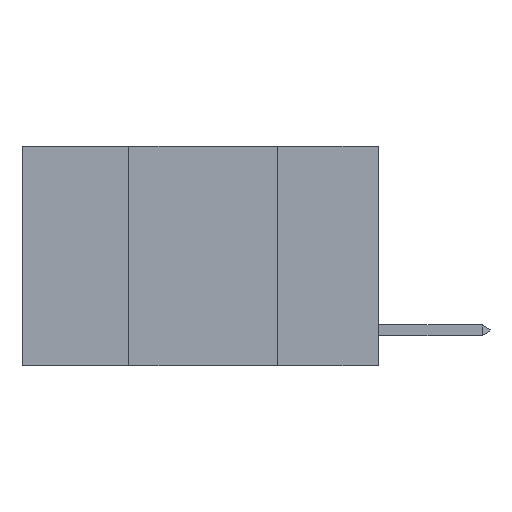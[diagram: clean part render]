
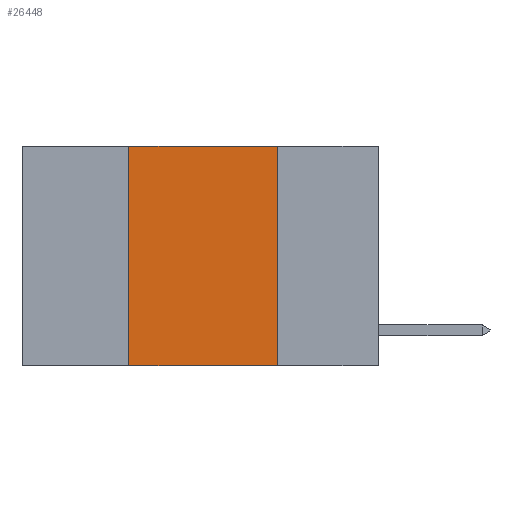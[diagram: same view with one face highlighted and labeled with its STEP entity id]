
A CAD part, left-side view. The second image highlights one B-rep face of the part: STEP entity #26448.
In plain terms, the highlighted planar face has unit normal (-1, 0, 0).
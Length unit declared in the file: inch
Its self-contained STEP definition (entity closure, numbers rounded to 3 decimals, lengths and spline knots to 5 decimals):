
#1099 = DIRECTION ( 'NONE',  ( 0., 0., -1. ) ) ;
#2393 = VERTEX_POINT ( 'NONE', #9922 ) ;
#3205 = CARTESIAN_POINT ( 'NONE',  ( 0., 0.17, -0.37 ) ) ;
#3824 = EDGE_CURVE ( 'NONE', #16245, #5316, #20547, .T. ) ;
#4084 = ORIENTED_EDGE ( 'NONE', *, *, #19276, .F. ) ;
#5316 = VERTEX_POINT ( 'NONE', #27220 ) ;
#5476 = ORIENTED_EDGE ( 'NONE', *, *, #18995, .T. ) ;
#6569 = CARTESIAN_POINT ( 'NONE',  ( 0., 0.42, 0. ) ) ;
#9922 = CARTESIAN_POINT ( 'NONE',  ( 0., 0.42, -0.37 ) ) ;
#10501 = EDGE_LOOP ( 'NONE', ( #4084, #27363, #22295, #5476 ) ) ;
#10822 = VECTOR ( 'NONE', #13448, 39.37008 ) ;
#11763 = CARTESIAN_POINT ( 'NONE',  ( 0., 0.6, 0. ) ) ;
#13448 = DIRECTION ( 'NONE',  ( 0., -1., 0. ) ) ;
#13741 = DIRECTION ( 'NONE',  ( 0., -1., 0. ) ) ;
#14015 = DIRECTION ( 'NONE',  ( 0., 0., -1. ) ) ;
#15654 = VECTOR ( 'NONE', #1099, 39.37008 ) ;
#16245 = VERTEX_POINT ( 'NONE', #17570 ) ;
#17015 = LINE ( 'NONE', #27381, #15654 ) ;
#17368 = LINE ( 'NONE', #24267, #10822 ) ;
#17570 = CARTESIAN_POINT ( 'NONE',  ( 0., 0.42, 0. ) ) ;
#18064 = VECTOR ( 'NONE', #24081, 39.37008 ) ;
#18582 = VERTEX_POINT ( 'NONE', #3205 ) ;
#18942 = EDGE_CURVE ( 'NONE', #2393, #16245, #24495, .T. ) ;
#18995 = EDGE_CURVE ( 'NONE', #2393, #18582, #17368, .T. ) ;
#19276 = EDGE_CURVE ( 'NONE', #5316, #18582, #17015, .T. ) ;
#20547 = LINE ( 'NONE', #26736, #26981 ) ;
#22295 = ORIENTED_EDGE ( 'NONE', *, *, #18942, .F. ) ;
#22309 = FACE_OUTER_BOUND ( 'NONE', #10501, .T. ) ;
#24081 = DIRECTION ( 'NONE',  ( 0., 0., 1. ) ) ;
#24267 = CARTESIAN_POINT ( 'NONE',  ( 0., 0.6, -0.37 ) ) ;
#24495 = LINE ( 'NONE', #6569, #18064 ) ;
#24817 = PLANE ( 'NONE',  #28280 ) ;
#26448 = ADVANCED_FACE ( 'NONE', ( #22309 ), #24817, .F. ) ;
#26736 = CARTESIAN_POINT ( 'NONE',  ( 0., 0.6, 0. ) ) ;
#26981 = VECTOR ( 'NONE', #13741, 39.37008 ) ;
#26996 = DIRECTION ( 'NONE',  ( 1., 0., 0. ) ) ;
#27220 = CARTESIAN_POINT ( 'NONE',  ( 0., 0.17, 0. ) ) ;
#27363 = ORIENTED_EDGE ( 'NONE', *, *, #3824, .F. ) ;
#27381 = CARTESIAN_POINT ( 'NONE',  ( 0., 0.17, 0. ) ) ;
#28280 = AXIS2_PLACEMENT_3D ( 'NONE', #11763, #26996, #14015 ) ;
